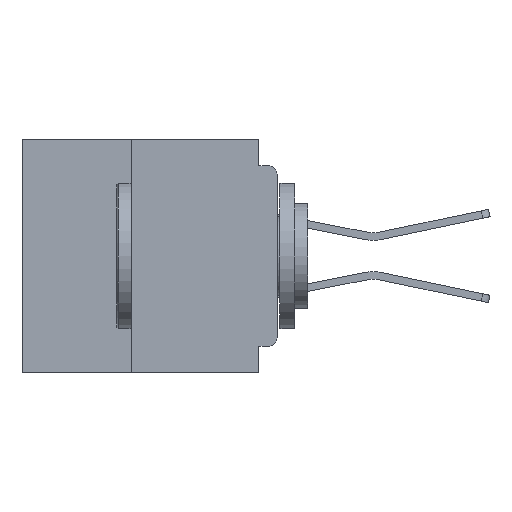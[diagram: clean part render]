
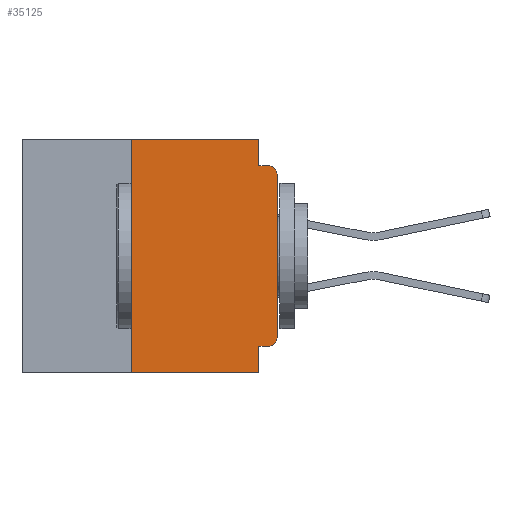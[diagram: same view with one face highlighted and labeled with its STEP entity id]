
A CAD part, left-side view. The second image highlights one B-rep face of the part: STEP entity #35125.
In plain terms, the highlighted planar face has unit normal (-1, 0, 0).
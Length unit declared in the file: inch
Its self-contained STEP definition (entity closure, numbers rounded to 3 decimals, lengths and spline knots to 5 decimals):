
#807 = EDGE_CURVE ( 'NONE', #9064, #27283, #13177, .T. ) ;
#1266 = VERTEX_POINT ( 'NONE', #21708 ) ;
#2110 = EDGE_LOOP ( 'NONE', ( #25730, #25800, #25868, #27550, #27581, #28067, #28176, #30778, #30821, #32042 ) ) ;
#2118 = AXIS2_PLACEMENT_3D ( 'NONE', #33082, #15616, #35935 ) ;
#2619 = CARTESIAN_POINT ( 'NONE',  ( 0., 0.015, -0.06 ) ) ;
#3242 = CARTESIAN_POINT ( 'NONE',  ( 0., 0., -0.06 ) ) ;
#3570 = DIRECTION ( 'NONE',  ( 0., -1., 0. ) ) ;
#3760 = VERTEX_POINT ( 'NONE', #28102 ) ;
#3809 = FACE_OUTER_BOUND ( 'NONE', #2110, .T. ) ;
#5663 = DIRECTION ( 'NONE',  ( 0., 0., -1. ) ) ;
#6006 = AXIS2_PLACEMENT_3D ( 'NONE', #2619, #23359, #5663 ) ;
#6141 = CARTESIAN_POINT ( 'NONE',  ( 0., 0.015, -0.045 ) ) ;
#6389 = CARTESIAN_POINT ( 'NONE',  ( 0., 0., -0.045 ) ) ;
#6606 = PLANE ( 'NONE',  #2118 ) ;
#7169 = CIRCLE ( 'NONE', #6006, 0.015 ) ;
#8989 = EDGE_CURVE ( 'NONE', #29959, #14999, #10312, .T. ) ;
#9032 = VECTOR ( 'NONE', #35723, 39.37008 ) ;
#9064 = VERTEX_POINT ( 'NONE', #30765 ) ;
#9367 = VERTEX_POINT ( 'NONE', #6141 ) ;
#9485 = EDGE_CURVE ( 'NONE', #14999, #23607, #37571, .T. ) ;
#9893 = VECTOR ( 'NONE', #15863, 39.37008 ) ;
#9912 = EDGE_CURVE ( 'NONE', #1266, #26439, #24992, .T. ) ;
#10312 = LINE ( 'NONE', #33303, #17262 ) ;
#11448 = CARTESIAN_POINT ( 'NONE',  ( 0., 0.031, -0.4 ) ) ;
#13177 = LINE ( 'NONE', #30430, #35470 ) ;
#13199 = CARTESIAN_POINT ( 'NONE',  ( 0., 0.25, -0.4 ) ) ;
#13764 = CARTESIAN_POINT ( 'NONE',  ( 0., 0.015, -0.34 ) ) ;
#14513 = EDGE_CURVE ( 'NONE', #9064, #1266, #30831, .T. ) ;
#14999 = VERTEX_POINT ( 'NONE', #18809 ) ;
#15616 = DIRECTION ( 'NONE',  ( 1., 0., 0. ) ) ;
#15787 = DIRECTION ( 'NONE',  ( 0., -1., 0. ) ) ;
#15810 = EDGE_CURVE ( 'NONE', #27283, #17126, #21970, .T. ) ;
#15855 = EDGE_CURVE ( 'NONE', #26439, #9367, #7169, .T. ) ;
#15863 = DIRECTION ( 'NONE',  ( 0., 0., -1. ) ) ;
#16702 = DIRECTION ( 'NONE',  ( 0., 0., -1. ) ) ;
#17126 = VERTEX_POINT ( 'NONE', #31979 ) ;
#17195 = VECTOR ( 'NONE', #20591, 39.37008 ) ;
#17262 = VECTOR ( 'NONE', #27436, 39.37008 ) ;
#18398 = CARTESIAN_POINT ( 'NONE',  ( 0., 0.437, -0.4 ) ) ;
#18642 = CARTESIAN_POINT ( 'NONE',  ( 0., 0.031, 0. ) ) ;
#18676 = LINE ( 'NONE', #18642, #9893 ) ;
#18809 = CARTESIAN_POINT ( 'NONE',  ( 0., 0.25, 0. ) ) ;
#19681 = CARTESIAN_POINT ( 'NONE',  ( 0., 0.031, 0. ) ) ;
#20591 = DIRECTION ( 'NONE',  ( 0., 0., 1. ) ) ;
#21708 = CARTESIAN_POINT ( 'NONE',  ( 0., 0., -0.34 ) ) ;
#21970 = LINE ( 'NONE', #11448, #37318 ) ;
#23359 = DIRECTION ( 'NONE',  ( -1., 0., 0. ) ) ;
#23543 = AXIS2_PLACEMENT_3D ( 'NONE', #13764, #34168, #16702 ) ;
#23607 = VERTEX_POINT ( 'NONE', #19681 ) ;
#24485 = CARTESIAN_POINT ( 'NONE',  ( 0., 0.437, 0. ) ) ;
#24992 = LINE ( 'NONE', #37856, #17195 ) ;
#25730 = ORIENTED_EDGE ( 'NONE', *, *, #9912, .T. ) ;
#25800 = ORIENTED_EDGE ( 'NONE', *, *, #15855, .T. ) ;
#25868 = ORIENTED_EDGE ( 'NONE', *, *, #34436, .F. ) ;
#26439 = VERTEX_POINT ( 'NONE', #3242 ) ;
#27283 = VERTEX_POINT ( 'NONE', #34356 ) ;
#27436 = DIRECTION ( 'NONE',  ( 0., 0., 1. ) ) ;
#27550 = ORIENTED_EDGE ( 'NONE', *, *, #35171, .F. ) ;
#27581 = ORIENTED_EDGE ( 'NONE', *, *, #9485, .F. ) ;
#28067 = ORIENTED_EDGE ( 'NONE', *, *, #8989, .F. ) ;
#28102 = CARTESIAN_POINT ( 'NONE',  ( 0., 0.031, -0.045 ) ) ;
#28176 = ORIENTED_EDGE ( 'NONE', *, *, #32672, .T. ) ;
#29959 = VERTEX_POINT ( 'NONE', #13199 ) ;
#30430 = CARTESIAN_POINT ( 'NONE',  ( 0., 0., -0.355 ) ) ;
#30687 = DIRECTION ( 'NONE',  ( 0., 1., 0. ) ) ;
#30765 = CARTESIAN_POINT ( 'NONE',  ( 0., 0.015, -0.355 ) ) ;
#30778 = ORIENTED_EDGE ( 'NONE', *, *, #15810, .F. ) ;
#30821 = ORIENTED_EDGE ( 'NONE', *, *, #807, .F. ) ;
#30831 = CIRCLE ( 'NONE', #23543, 0.015 ) ;
#30952 = VECTOR ( 'NONE', #15787, 39.37008 ) ;
#31705 = VECTOR ( 'NONE', #3570, 39.37008 ) ;
#31929 = DIRECTION ( 'NONE',  ( 0., 0., -1. ) ) ;
#31979 = CARTESIAN_POINT ( 'NONE',  ( 0., 0.031, -0.4 ) ) ;
#32042 = ORIENTED_EDGE ( 'NONE', *, *, #14513, .T. ) ;
#32614 = LINE ( 'NONE', #18398, #31705 ) ;
#32672 = EDGE_CURVE ( 'NONE', #29959, #17126, #32614, .T. ) ;
#33082 = CARTESIAN_POINT ( 'NONE',  ( 0., 0.437, 0. ) ) ;
#33303 = CARTESIAN_POINT ( 'NONE',  ( 0., 0.25, -0.4 ) ) ;
#34168 = DIRECTION ( 'NONE',  ( -1., 0., 0. ) ) ;
#34356 = CARTESIAN_POINT ( 'NONE',  ( 0., 0.031, -0.355 ) ) ;
#34436 = EDGE_CURVE ( 'NONE', #3760, #9367, #37295, .T. ) ;
#35125 = ADVANCED_FACE ( 'NONE', ( #3809 ), #6606, .F. ) ;
#35171 = EDGE_CURVE ( 'NONE', #23607, #3760, #18676, .T. ) ;
#35470 = VECTOR ( 'NONE', #30687, 39.37008 ) ;
#35723 = DIRECTION ( 'NONE',  ( 0., -1., 0. ) ) ;
#35935 = DIRECTION ( 'NONE',  ( 0., 0., -1. ) ) ;
#37295 = LINE ( 'NONE', #6389, #9032 ) ;
#37318 = VECTOR ( 'NONE', #31929, 39.37008 ) ;
#37571 = LINE ( 'NONE', #24485, #30952 ) ;
#37856 = CARTESIAN_POINT ( 'NONE',  ( 0., 0., 0. ) ) ;
